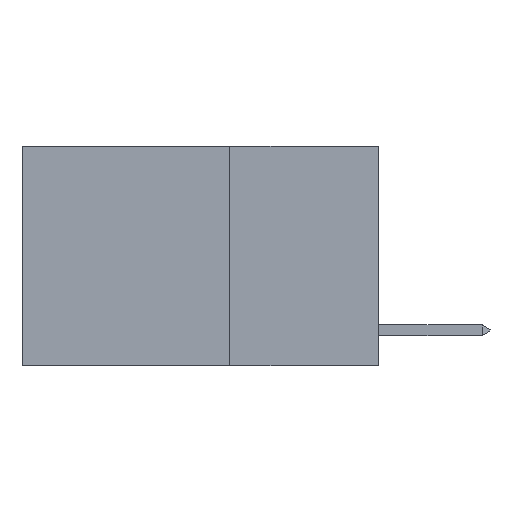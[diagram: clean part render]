
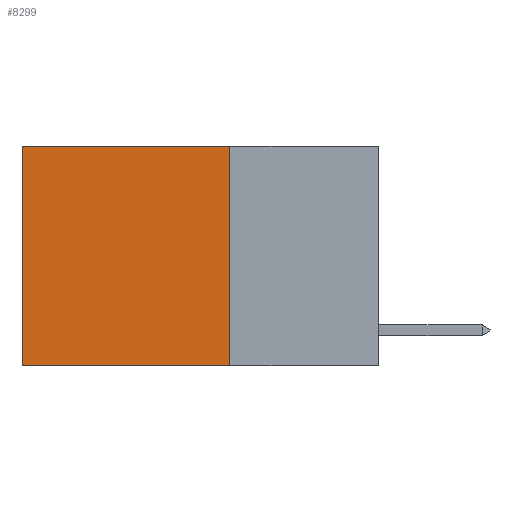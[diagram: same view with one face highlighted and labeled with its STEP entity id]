
A CAD part, left-side view. The second image highlights one B-rep face of the part: STEP entity #8299.
In plain terms, the highlighted planar face has unit normal (-1, 0, 0).
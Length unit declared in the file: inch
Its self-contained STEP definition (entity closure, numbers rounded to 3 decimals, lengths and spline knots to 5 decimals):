
#25 = VERTEX_POINT ( 'NONE', #5051 ) ;
#304 = VERTEX_POINT ( 'NONE', #1772 ) ;
#1772 = CARTESIAN_POINT ( 'NONE',  ( 0.2625, 0.25, 0. ) ) ;
#1838 = LINE ( 'NONE', #9584, #10822 ) ;
#2109 = EDGE_LOOP ( 'NONE', ( #6699, #3413, #3757, #9438 ) ) ;
#2407 = CARTESIAN_POINT ( 'NONE',  ( 0.2625, 0.25, 0. ) ) ;
#2621 = DIRECTION ( 'NONE',  ( 0., 1., 0. ) ) ;
#3340 = LINE ( 'NONE', #2407, #7764 ) ;
#3413 = ORIENTED_EDGE ( 'NONE', *, *, #3668, .F. ) ;
#3668 = EDGE_CURVE ( 'NONE', #25, #5274, #8557, .T. ) ;
#3757 = ORIENTED_EDGE ( 'NONE', *, *, #3769, .F. ) ;
#3769 = EDGE_CURVE ( 'NONE', #304, #25, #3340, .T. ) ;
#4137 = CARTESIAN_POINT ( 'NONE',  ( 0.2625, 0.6, 0. ) ) ;
#4930 = DIRECTION ( 'NONE',  ( 0., 0., -1. ) ) ;
#4984 = VECTOR ( 'NONE', #5026, 39.37008 ) ;
#5026 = DIRECTION ( 'NONE',  ( 0., 0., -1. ) ) ;
#5051 = CARTESIAN_POINT ( 'NONE',  ( 0.2625, 0.25, -0.37 ) ) ;
#5274 = VERTEX_POINT ( 'NONE', #5618 ) ;
#5618 = CARTESIAN_POINT ( 'NONE',  ( 0.2625, 0.6, -0.37 ) ) ;
#5789 = CARTESIAN_POINT ( 'NONE',  ( 0.2625, 0.25, 0. ) ) ;
#6372 = EDGE_CURVE ( 'NONE', #304, #9590, #1838, .T. ) ;
#6611 = CARTESIAN_POINT ( 'NONE',  ( 0.2625, 0.25, -0.37 ) ) ;
#6699 = ORIENTED_EDGE ( 'NONE', *, *, #8966, .T. ) ;
#7457 = FACE_OUTER_BOUND ( 'NONE', #2109, .T. ) ;
#7521 = PLANE ( 'NONE',  #10901 ) ;
#7764 = VECTOR ( 'NONE', #8614, 39.37008 ) ;
#8299 = ADVANCED_FACE ( 'NONE', ( #7457 ), #7521, .F. ) ;
#8312 = VECTOR ( 'NONE', #9198, 39.37008 ) ;
#8557 = LINE ( 'NONE', #6611, #8312 ) ;
#8614 = DIRECTION ( 'NONE',  ( 0., 0., -1. ) ) ;
#8966 = EDGE_CURVE ( 'NONE', #9590, #5274, #9785, .T. ) ;
#9198 = DIRECTION ( 'NONE',  ( 0., 1., 0. ) ) ;
#9438 = ORIENTED_EDGE ( 'NONE', *, *, #6372, .T. ) ;
#9584 = CARTESIAN_POINT ( 'NONE',  ( 0.2625, 0.25, 0. ) ) ;
#9590 = VERTEX_POINT ( 'NONE', #10969 ) ;
#9785 = LINE ( 'NONE', #4137, #4984 ) ;
#10020 = DIRECTION ( 'NONE',  ( 1., 0., 0. ) ) ;
#10822 = VECTOR ( 'NONE', #2621, 39.37008 ) ;
#10901 = AXIS2_PLACEMENT_3D ( 'NONE', #5789, #10020, #4930 ) ;
#10969 = CARTESIAN_POINT ( 'NONE',  ( 0.2625, 0.6, 0. ) ) ;
